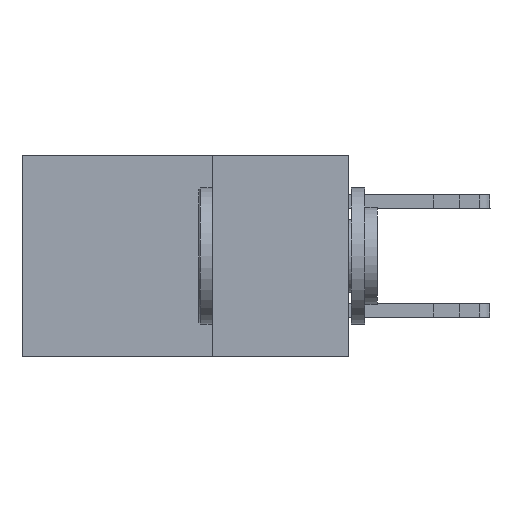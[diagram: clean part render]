
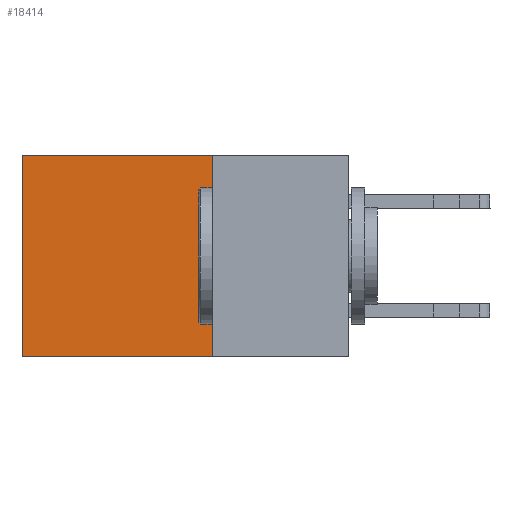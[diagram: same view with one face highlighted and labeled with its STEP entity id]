
A CAD part, left-side view. The second image highlights one B-rep face of the part: STEP entity #18414.
In plain terms, the highlighted planar face has unit normal (-1, 0, 0).
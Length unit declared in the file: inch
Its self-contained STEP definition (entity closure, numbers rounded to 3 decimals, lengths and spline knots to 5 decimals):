
#2441 = VERTEX_POINT ( 'NONE', #17364 ) ;
#3407 = EDGE_CURVE ( 'NONE', #18693, #21521, #8881, .T. ) ;
#3462 = DIRECTION ( 'NONE',  ( 0., 1., 0. ) ) ;
#3986 = DIRECTION ( 'NONE',  ( 0., 0., -1. ) ) ;
#4154 = CARTESIAN_POINT ( 'NONE',  ( 0.2615, 0.25, -0.37 ) ) ;
#5870 = AXIS2_PLACEMENT_3D ( 'NONE', #9223, #16174, #12959 ) ;
#6273 = LINE ( 'NONE', #4154, #21513 ) ;
#6955 = LINE ( 'NONE', #10472, #10598 ) ;
#7241 = VERTEX_POINT ( 'NONE', #13135 ) ;
#7820 = CARTESIAN_POINT ( 'NONE',  ( 0.2615, 0.25, -0.37 ) ) ;
#7985 = EDGE_LOOP ( 'NONE', ( #19004, #14243, #9858, #10631 ) ) ;
#8136 = CARTESIAN_POINT ( 'NONE',  ( 0.2615, 0.6, 0. ) ) ;
#8881 = LINE ( 'NONE', #19147, #20244 ) ;
#9223 = CARTESIAN_POINT ( 'NONE',  ( 0.2615, 0.25, -0.37 ) ) ;
#9858 = ORIENTED_EDGE ( 'NONE', *, *, #20318, .F. ) ;
#10472 = CARTESIAN_POINT ( 'NONE',  ( 0.2615, 0.6, -0.37 ) ) ;
#10598 = VECTOR ( 'NONE', #13887, 39.37008 ) ;
#10631 = ORIENTED_EDGE ( 'NONE', *, *, #3407, .T. ) ;
#12959 = DIRECTION ( 'NONE',  ( 0., 0., -1. ) ) ;
#13135 = CARTESIAN_POINT ( 'NONE',  ( 0.2615, 0.6, -0.37 ) ) ;
#13887 = DIRECTION ( 'NONE',  ( 0., 0., -1. ) ) ;
#14243 = ORIENTED_EDGE ( 'NONE', *, *, #18061, .F. ) ;
#14666 = FACE_OUTER_BOUND ( 'NONE', #7985, .T. ) ;
#16174 = DIRECTION ( 'NONE',  ( 1., 0., 0. ) ) ;
#17364 = CARTESIAN_POINT ( 'NONE',  ( 0.2615, 0.25, -0.37 ) ) ;
#17909 = DIRECTION ( 'NONE',  ( 0., 1., 0. ) ) ;
#18061 = EDGE_CURVE ( 'NONE', #2441, #7241, #6273, .T. ) ;
#18317 = EDGE_CURVE ( 'NONE', #21521, #7241, #6955, .T. ) ;
#18414 = ADVANCED_FACE ( 'NONE', ( #14666 ), #21307, .F. ) ;
#18693 = VERTEX_POINT ( 'NONE', #19343 ) ;
#19004 = ORIENTED_EDGE ( 'NONE', *, *, #18317, .T. ) ;
#19027 = VECTOR ( 'NONE', #3986, 39.37008 ) ;
#19147 = CARTESIAN_POINT ( 'NONE',  ( 0.2615, 0.25, 0. ) ) ;
#19343 = CARTESIAN_POINT ( 'NONE',  ( 0.2615, 0.25, 0. ) ) ;
#20244 = VECTOR ( 'NONE', #3462, 39.37008 ) ;
#20318 = EDGE_CURVE ( 'NONE', #18693, #2441, #21846, .T. ) ;
#21307 = PLANE ( 'NONE',  #5870 ) ;
#21513 = VECTOR ( 'NONE', #17909, 39.37008 ) ;
#21521 = VERTEX_POINT ( 'NONE', #8136 ) ;
#21846 = LINE ( 'NONE', #7820, #19027 ) ;
